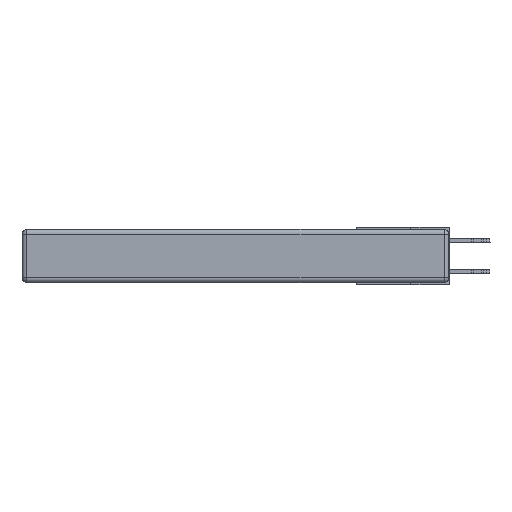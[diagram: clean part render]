
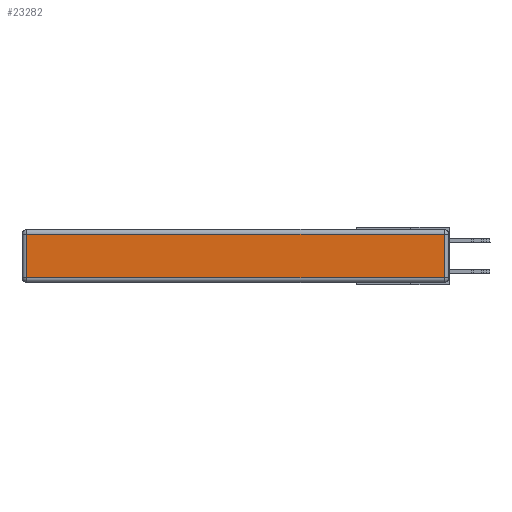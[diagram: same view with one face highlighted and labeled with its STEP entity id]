
A CAD part, left-side view. The second image highlights one B-rep face of the part: STEP entity #23282.
In plain terms, the highlighted planar face has unit normal (-1, 0, 0).
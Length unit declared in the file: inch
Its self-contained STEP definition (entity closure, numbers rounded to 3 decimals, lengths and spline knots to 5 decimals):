
#1247 = AXIS2_PLACEMENT_3D ( 'NONE', #2087, #25575, #9645 ) ;
#1994 = VERTEX_POINT ( 'NONE', #17490 ) ;
#2087 = CARTESIAN_POINT ( 'NONE',  ( 0., 0., -0.343 ) ) ;
#2537 = LINE ( 'NONE', #5232, #29726 ) ;
#5232 = CARTESIAN_POINT ( 'NONE',  ( 0., 0., -0.313 ) ) ;
#6115 = VERTEX_POINT ( 'NONE', #24558 ) ;
#6488 = VERTEX_POINT ( 'NONE', #7159 ) ;
#6762 = CARTESIAN_POINT ( 'NONE',  ( 0., 2.75, -0.03 ) ) ;
#7038 = VERTEX_POINT ( 'NONE', #26462 ) ;
#7159 = CARTESIAN_POINT ( 'NONE',  ( 0., 0.03, -0.313 ) ) ;
#9317 = VECTOR ( 'NONE', #25455, 39.37008 ) ;
#9645 = DIRECTION ( 'NONE',  ( 0., 0., 1. ) ) ;
#11884 = ORIENTED_EDGE ( 'NONE', *, *, #19264, .T. ) ;
#12084 = VECTOR ( 'NONE', #28757, 39.37008 ) ;
#12310 = ORIENTED_EDGE ( 'NONE', *, *, #30316, .T. ) ;
#12589 = CARTESIAN_POINT ( 'NONE',  ( 0., 2.72, -0.343 ) ) ;
#15556 = EDGE_CURVE ( 'NONE', #7038, #1994, #17893, .T. ) ;
#15816 = VECTOR ( 'NONE', #22652, 39.37008 ) ;
#15943 = DIRECTION ( 'NONE',  ( 0., -1., 0. ) ) ;
#17490 = CARTESIAN_POINT ( 'NONE',  ( 0., 2.72, -0.03 ) ) ;
#17893 = LINE ( 'NONE', #6762, #15816 ) ;
#19264 = EDGE_CURVE ( 'NONE', #6115, #6488, #2537, .T. ) ;
#20890 = ORIENTED_EDGE ( 'NONE', *, *, #15556, .T. ) ;
#22257 = ORIENTED_EDGE ( 'NONE', *, *, #26667, .T. ) ;
#22652 = DIRECTION ( 'NONE',  ( 0., 1., 0. ) ) ;
#23282 = ADVANCED_FACE ( 'NONE', ( #23764 ), #31430, .T. ) ;
#23764 = FACE_OUTER_BOUND ( 'NONE', #27567, .T. ) ;
#24271 = LINE ( 'NONE', #12589, #12084 ) ;
#24558 = CARTESIAN_POINT ( 'NONE',  ( 0., 2.72, -0.313 ) ) ;
#25455 = DIRECTION ( 'NONE',  ( 0., 0., 1. ) ) ;
#25575 = DIRECTION ( 'NONE',  ( -1., 0., 0. ) ) ;
#26462 = CARTESIAN_POINT ( 'NONE',  ( 0., 0.03, -0.03 ) ) ;
#26667 = EDGE_CURVE ( 'NONE', #6488, #7038, #30263, .T. ) ;
#27567 = EDGE_LOOP ( 'NONE', ( #11884, #22257, #20890, #12310 ) ) ;
#27948 = CARTESIAN_POINT ( 'NONE',  ( 0., 0.03, -0.343 ) ) ;
#28757 = DIRECTION ( 'NONE',  ( 0., 0., -1. ) ) ;
#29726 = VECTOR ( 'NONE', #15943, 39.37008 ) ;
#30263 = LINE ( 'NONE', #27948, #9317 ) ;
#30316 = EDGE_CURVE ( 'NONE', #1994, #6115, #24271, .T. ) ;
#31430 = PLANE ( 'NONE',  #1247 ) ;
